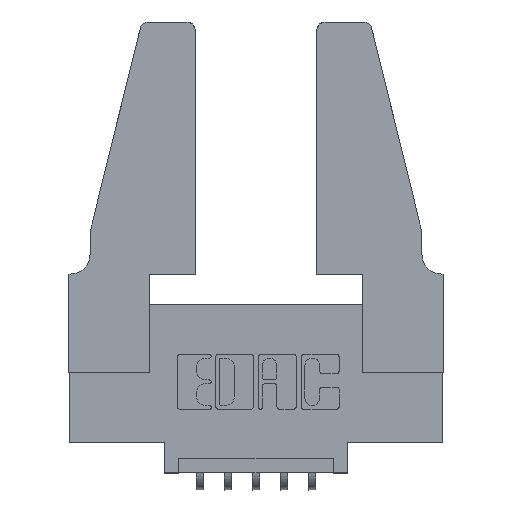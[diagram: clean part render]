
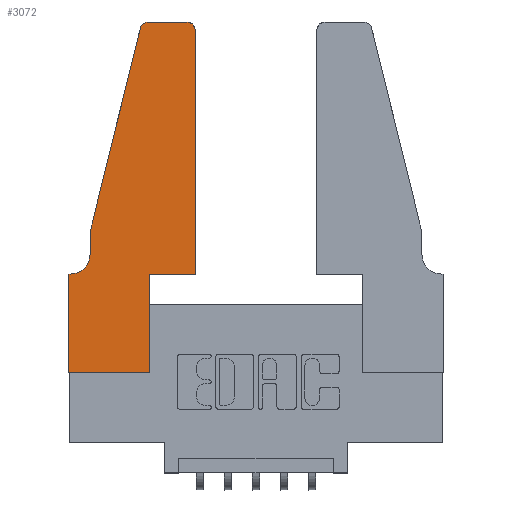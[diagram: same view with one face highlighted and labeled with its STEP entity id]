
A CAD part, top view. The second image highlights one B-rep face of the part: STEP entity #3072.
In plain terms, the highlighted planar face has unit normal (0, 0, 1).
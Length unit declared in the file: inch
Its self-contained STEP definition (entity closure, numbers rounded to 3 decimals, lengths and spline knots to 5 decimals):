
#1 = EDGE_CURVE ( 'NONE', #6292, #7039, #6388, .T. ) ;
#111 = VERTEX_POINT ( 'NONE', #704 ) ;
#174 = CARTESIAN_POINT ( 'NONE',  ( 0.4505, 1.22, 0.37 ) ) ;
#416 = DIRECTION ( 'NONE',  ( -1., 0., 0. ) ) ;
#507 = VECTOR ( 'NONE', #7361, 39.37008 ) ;
#685 = ORIENTED_EDGE ( 'NONE', *, *, #5903, .T. ) ;
#704 = CARTESIAN_POINT ( 'NONE',  ( 0., 0.35, 0.37 ) ) ;
#756 = LINE ( 'NONE', #10914, #9094 ) ;
#771 = VERTEX_POINT ( 'NONE', #3717 ) ;
#791 = ORIENTED_EDGE ( 'NONE', *, *, #5286, .T. ) ;
#897 = VECTOR ( 'NONE', #8679, 39.37008 ) ;
#1011 = EDGE_CURVE ( 'NONE', #6572, #5166, #756, .T. ) ;
#1048 = DIRECTION ( 'NONE',  ( -1., 0., 0. ) ) ;
#1160 = CARTESIAN_POINT ( 'NONE',  ( 0.0755, 0.35, 0.37 ) ) ;
#1275 = CARTESIAN_POINT ( 'NONE',  ( 0.0755, 0.5, 0.37 ) ) ;
#1631 = AXIS2_PLACEMENT_3D ( 'NONE', #7691, #1790, #5997 ) ;
#1738 = ORIENTED_EDGE ( 'NONE', *, *, #11027, .T. ) ;
#1770 = CARTESIAN_POINT ( 'NONE',  ( 0., 0., 0.37 ) ) ;
#1790 = DIRECTION ( 'NONE',  ( 0., 0., 1. ) ) ;
#1812 = DIRECTION ( 'NONE',  ( 1., 0., 0. ) ) ;
#2055 = LINE ( 'NONE', #9670, #10904 ) ;
#2077 = DIRECTION ( 'NONE',  ( 0., 0., 1. ) ) ;
#2187 = CARTESIAN_POINT ( 'NONE',  ( 0.2865, 0.35, 0.37 ) ) ;
#2201 = VECTOR ( 'NONE', #1048, 39.37008 ) ;
#2293 = EDGE_CURVE ( 'NONE', #3898, #3856, #3323, .T. ) ;
#2347 = VECTOR ( 'NONE', #8600, 39.37008 ) ;
#2356 = FACE_OUTER_BOUND ( 'NONE', #9080, .T. ) ;
#2531 = VERTEX_POINT ( 'NONE', #7486 ) ;
#2551 = DIRECTION ( 'NONE',  ( 0., 1., 0. ) ) ;
#2706 = CARTESIAN_POINT ( 'NONE',  ( 0., 0., 0.37 ) ) ;
#2900 = DIRECTION ( 'NONE',  ( 0., 0., -1. ) ) ;
#3072 = ADVANCED_FACE ( 'NONE', ( #2356 ), #8935, .T. ) ;
#3112 = EDGE_CURVE ( 'NONE', #5166, #5839, #6208, .T. ) ;
#3144 = DIRECTION ( 'NONE',  ( -0.239, -0.971, 0. ) ) ;
#3323 = LINE ( 'NONE', #8506, #7032 ) ;
#3387 = ORIENTED_EDGE ( 'NONE', *, *, #3112, .T. ) ;
#3717 = CARTESIAN_POINT ( 'NONE',  ( 0.0055, 0.35, 0.37 ) ) ;
#3738 = LINE ( 'NONE', #2706, #897 ) ;
#3804 = DIRECTION ( 'NONE',  ( 1., 0., 0. ) ) ;
#3806 = CARTESIAN_POINT ( 'NONE',  ( 0., 0.35, 0.37 ) ) ;
#3856 = VERTEX_POINT ( 'NONE', #174 ) ;
#3898 = VERTEX_POINT ( 'NONE', #8588 ) ;
#3996 = CARTESIAN_POINT ( 'NONE',  ( 0.4505, 0.35, 0.37 ) ) ;
#4055 = EDGE_CURVE ( 'NONE', #7039, #3898, #6469, .T. ) ;
#4104 = AXIS2_PLACEMENT_3D ( 'NONE', #7169, #2077, #3804 ) ;
#4310 = LINE ( 'NONE', #10486, #5098 ) ;
#4458 = LINE ( 'NONE', #1160, #2201 ) ;
#4652 = CARTESIAN_POINT ( 'NONE',  ( 0.0055, 0.42, 0.37 ) ) ;
#4807 = VERTEX_POINT ( 'NONE', #5298 ) ;
#4818 = EDGE_CURVE ( 'NONE', #771, #111, #4458, .T. ) ;
#4825 = ORIENTED_EDGE ( 'NONE', *, *, #1, .T. ) ;
#5098 = VECTOR ( 'NONE', #1812, 39.37008 ) ;
#5166 = VERTEX_POINT ( 'NONE', #6535 ) ;
#5239 = ORIENTED_EDGE ( 'NONE', *, *, #2293, .T. ) ;
#5266 = EDGE_CURVE ( 'NONE', #4807, #2531, #2055, .T. ) ;
#5286 = EDGE_CURVE ( 'NONE', #6490, #6292, #4310, .T. ) ;
#5298 = CARTESIAN_POINT ( 'NONE',  ( 0.4205, 1.25, 0.37 ) ) ;
#5393 = ORIENTED_EDGE ( 'NONE', *, *, #7966, .T. ) ;
#5673 = EDGE_CURVE ( 'NONE', #2531, #6572, #10114, .T. ) ;
#5839 = VERTEX_POINT ( 'NONE', #10506 ) ;
#5903 = EDGE_CURVE ( 'NONE', #5839, #771, #9994, .T. ) ;
#5997 = DIRECTION ( 'NONE',  ( 1., 0., 0. ) ) ;
#6208 = LINE ( 'NONE', #1275, #10558 ) ;
#6283 = ORIENTED_EDGE ( 'NONE', *, *, #1011, .T. ) ;
#6291 = DIRECTION ( 'NONE',  ( 0., -1., 0. ) ) ;
#6292 = VERTEX_POINT ( 'NONE', #7715 ) ;
#6388 = LINE ( 'NONE', #2187, #507 ) ;
#6438 = AXIS2_PLACEMENT_3D ( 'NONE', #3806, #8170, #9828 ) ;
#6469 = LINE ( 'NONE', #3996, #2347 ) ;
#6490 = VERTEX_POINT ( 'NONE', #1770 ) ;
#6535 = CARTESIAN_POINT ( 'NONE',  ( 0.0755, 0.5, 0.37 ) ) ;
#6572 = VERTEX_POINT ( 'NONE', #10143 ) ;
#6995 = ORIENTED_EDGE ( 'NONE', *, *, #4055, .T. ) ;
#7032 = VECTOR ( 'NONE', #2551, 39.37008 ) ;
#7039 = VERTEX_POINT ( 'NONE', #10352 ) ;
#7169 = CARTESIAN_POINT ( 'NONE',  ( 0.4205, 1.22, 0.37 ) ) ;
#7241 = ORIENTED_EDGE ( 'NONE', *, *, #4818, .T. ) ;
#7361 = DIRECTION ( 'NONE',  ( 0., 1., 0. ) ) ;
#7486 = CARTESIAN_POINT ( 'NONE',  ( 0.284, 1.25, 0.37 ) ) ;
#7691 = CARTESIAN_POINT ( 'NONE',  ( 0.284, 1.22, 0.37 ) ) ;
#7715 = CARTESIAN_POINT ( 'NONE',  ( 0.2865, 0., 0.37 ) ) ;
#7966 = EDGE_CURVE ( 'NONE', #3856, #4807, #9949, .T. ) ;
#8170 = DIRECTION ( 'NONE',  ( 0., 0., 1. ) ) ;
#8252 = ORIENTED_EDGE ( 'NONE', *, *, #5673, .T. ) ;
#8506 = CARTESIAN_POINT ( 'NONE',  ( 0.4505, 0.35, 0.37 ) ) ;
#8588 = CARTESIAN_POINT ( 'NONE',  ( 0.4505, 0.35, 0.37 ) ) ;
#8600 = DIRECTION ( 'NONE',  ( 1., 0., 0. ) ) ;
#8679 = DIRECTION ( 'NONE',  ( 0., -1., 0. ) ) ;
#8935 = PLANE ( 'NONE',  #6438 ) ;
#9080 = EDGE_LOOP ( 'NONE', ( #10989, #8252, #6283, #3387, #685, #7241, #1738, #791, #4825, #6995, #5239, #5393 ) ) ;
#9094 = VECTOR ( 'NONE', #3144, 39.37008 ) ;
#9670 = CARTESIAN_POINT ( 'NONE',  ( 0.2605, 1.25, 0.37 ) ) ;
#9828 = DIRECTION ( 'NONE',  ( 1., 0., 0. ) ) ;
#9949 = CIRCLE ( 'NONE', #4104, 0.03 ) ;
#9994 = CIRCLE ( 'NONE', #10070, 0.07 ) ;
#10070 = AXIS2_PLACEMENT_3D ( 'NONE', #4652, #2900, #416 ) ;
#10114 = CIRCLE ( 'NONE', #1631, 0.03 ) ;
#10143 = CARTESIAN_POINT ( 'NONE',  ( 0.25487, 1.22718, 0.37 ) ) ;
#10352 = CARTESIAN_POINT ( 'NONE',  ( 0.2865, 0.35, 0.37 ) ) ;
#10372 = DIRECTION ( 'NONE',  ( -1., 0., 0. ) ) ;
#10486 = CARTESIAN_POINT ( 'NONE',  ( 0., 0., 0.37 ) ) ;
#10506 = CARTESIAN_POINT ( 'NONE',  ( 0.0755, 0.42, 0.37 ) ) ;
#10558 = VECTOR ( 'NONE', #6291, 39.37008 ) ;
#10904 = VECTOR ( 'NONE', #10372, 39.37008 ) ;
#10914 = CARTESIAN_POINT ( 'NONE',  ( 0.0755, 0.5, 0.37 ) ) ;
#10989 = ORIENTED_EDGE ( 'NONE', *, *, #5266, .T. ) ;
#11027 = EDGE_CURVE ( 'NONE', #111, #6490, #3738, .T. ) ;
